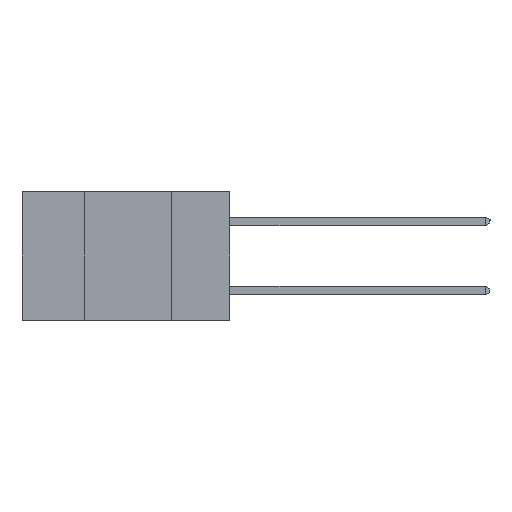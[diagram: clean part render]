
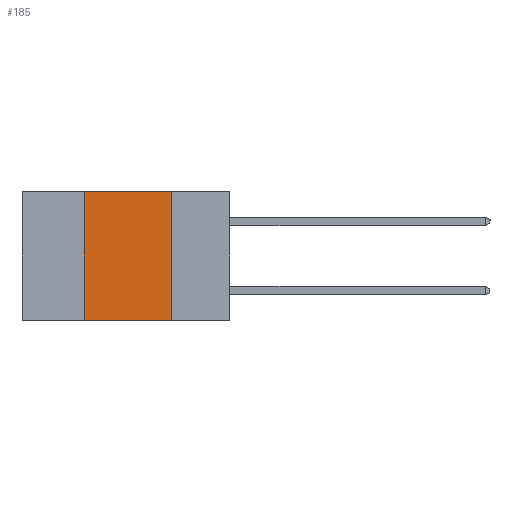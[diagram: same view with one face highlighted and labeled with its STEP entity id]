
A CAD part, left-side view. The second image highlights one B-rep face of the part: STEP entity #185.
In plain terms, the highlighted planar face has unit normal (-1, 0, 0).
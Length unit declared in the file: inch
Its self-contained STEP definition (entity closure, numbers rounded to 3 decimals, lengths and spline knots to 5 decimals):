
#153 = CARTESIAN_POINT ( 'NONE',  ( 0., 0.42, -0.37 ) ) ;
#185 = ADVANCED_FACE ( 'NONE', ( #3933 ), #5415, .F. ) ;
#1744 = CARTESIAN_POINT ( 'NONE',  ( 0., 0.6, 0. ) ) ;
#2353 = VERTEX_POINT ( 'NONE', #3241 ) ;
#2889 = DIRECTION ( 'NONE',  ( 0., 0., 1. ) ) ;
#2939 = CARTESIAN_POINT ( 'NONE',  ( 0., 0.6, 0. ) ) ;
#3241 = CARTESIAN_POINT ( 'NONE',  ( 0., 0.42, -0.37 ) ) ;
#3262 = LINE ( 'NONE', #8307, #6296 ) ;
#3490 = CARTESIAN_POINT ( 'NONE',  ( 0., 0.6, -0.37 ) ) ;
#3626 = EDGE_CURVE ( 'NONE', #2353, #8238, #10847, .T. ) ;
#3933 = FACE_OUTER_BOUND ( 'NONE', #14473, .T. ) ;
#4810 = DIRECTION ( 'NONE',  ( 0., -1., 0. ) ) ;
#4940 = VECTOR ( 'NONE', #2889, 39.37008 ) ;
#5152 = CARTESIAN_POINT ( 'NONE',  ( 0., 0.17, -0.37 ) ) ;
#5215 = LINE ( 'NONE', #1744, #12644 ) ;
#5415 = PLANE ( 'NONE',  #14108 ) ;
#6296 = VECTOR ( 'NONE', #13368, 39.37008 ) ;
#6434 = VERTEX_POINT ( 'NONE', #12619 ) ;
#6496 = DIRECTION ( 'NONE',  ( 1., 0., 0. ) ) ;
#6873 = ORIENTED_EDGE ( 'NONE', *, *, #3626, .T. ) ;
#8238 = VERTEX_POINT ( 'NONE', #5152 ) ;
#8307 = CARTESIAN_POINT ( 'NONE',  ( 0., 0.17, -0.37 ) ) ;
#8430 = ORIENTED_EDGE ( 'NONE', *, *, #15165, .F. ) ;
#9582 = CARTESIAN_POINT ( 'NONE',  ( 0., 0.17, 0. ) ) ;
#10079 = ORIENTED_EDGE ( 'NONE', *, *, #13822, .F. ) ;
#10847 = LINE ( 'NONE', #3490, #14529 ) ;
#12619 = CARTESIAN_POINT ( 'NONE',  ( 0., 0.42, 0. ) ) ;
#12644 = VECTOR ( 'NONE', #12837, 39.37008 ) ;
#12837 = DIRECTION ( 'NONE',  ( 0., -1., 0. ) ) ;
#13368 = DIRECTION ( 'NONE',  ( 0., 0., -1. ) ) ;
#13822 = EDGE_CURVE ( 'NONE', #6434, #15572, #5215, .T. ) ;
#14108 = AXIS2_PLACEMENT_3D ( 'NONE', #2939, #6496, #15523 ) ;
#14224 = LINE ( 'NONE', #153, #4940 ) ;
#14277 = EDGE_CURVE ( 'NONE', #2353, #6434, #14224, .T. ) ;
#14473 = EDGE_LOOP ( 'NONE', ( #8430, #10079, #15337, #6873 ) ) ;
#14529 = VECTOR ( 'NONE', #4810, 39.37008 ) ;
#15165 = EDGE_CURVE ( 'NONE', #15572, #8238, #3262, .T. ) ;
#15337 = ORIENTED_EDGE ( 'NONE', *, *, #14277, .F. ) ;
#15523 = DIRECTION ( 'NONE',  ( 0., 0., -1. ) ) ;
#15572 = VERTEX_POINT ( 'NONE', #9582 ) ;
